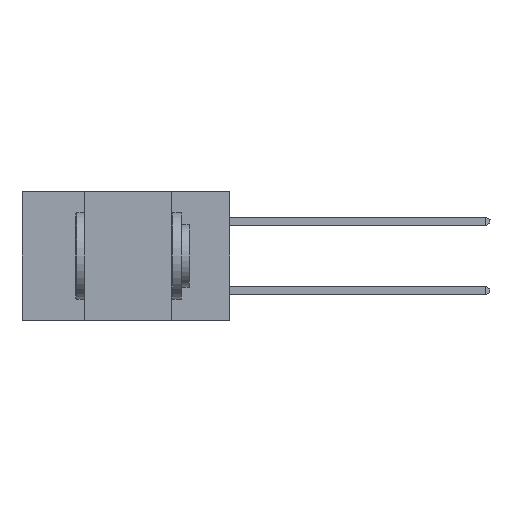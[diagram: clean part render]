
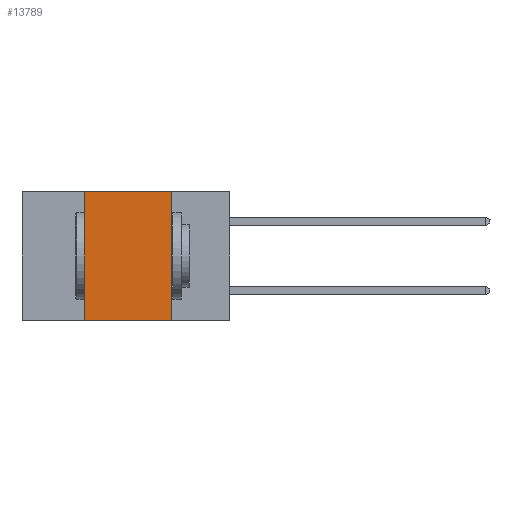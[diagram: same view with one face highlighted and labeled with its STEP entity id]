
A CAD part, left-side view. The second image highlights one B-rep face of the part: STEP entity #13789.
In plain terms, the highlighted planar face has unit normal (-1, 0, 0).
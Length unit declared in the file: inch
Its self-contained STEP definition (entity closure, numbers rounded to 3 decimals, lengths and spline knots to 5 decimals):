
#413 = EDGE_LOOP ( 'NONE', ( #3976, #6658, #12217, #16993 ) ) ;
#875 = LINE ( 'NONE', #3795, #2147 ) ;
#2047 = PLANE ( 'NONE',  #10269 ) ;
#2147 = VECTOR ( 'NONE', #11841, 39.37008 ) ;
#3258 = VERTEX_POINT ( 'NONE', #9242 ) ;
#3274 = CARTESIAN_POINT ( 'NONE',  ( 0., 0.6, 0. ) ) ;
#3795 = CARTESIAN_POINT ( 'NONE',  ( 0., 0.17, -0.37 ) ) ;
#3976 = ORIENTED_EDGE ( 'NONE', *, *, #6549, .F. ) ;
#5056 = EDGE_CURVE ( 'NONE', #7858, #17251, #11684, .T. ) ;
#5085 = VERTEX_POINT ( 'NONE', #14628 ) ;
#5785 = CARTESIAN_POINT ( 'NONE',  ( 0., 0.42, -0.37 ) ) ;
#6549 = EDGE_CURVE ( 'NONE', #17251, #5085, #875, .T. ) ;
#6658 = ORIENTED_EDGE ( 'NONE', *, *, #5056, .F. ) ;
#7161 = DIRECTION ( 'NONE',  ( 0., 0., 1. ) ) ;
#7631 = CARTESIAN_POINT ( 'NONE',  ( 0., 0.6, 0. ) ) ;
#7858 = VERTEX_POINT ( 'NONE', #12988 ) ;
#7904 = VECTOR ( 'NONE', #13191, 39.37008 ) ;
#8482 = VECTOR ( 'NONE', #10405, 39.37008 ) ;
#8838 = CARTESIAN_POINT ( 'NONE',  ( 0., 0.17, 0. ) ) ;
#9242 = CARTESIAN_POINT ( 'NONE',  ( 0., 0.42, -0.37 ) ) ;
#10114 = EDGE_CURVE ( 'NONE', #3258, #5085, #14468, .T. ) ;
#10263 = LINE ( 'NONE', #5785, #15673 ) ;
#10269 = AXIS2_PLACEMENT_3D ( 'NONE', #7631, #15756, #11819 ) ;
#10405 = DIRECTION ( 'NONE',  ( 0., -1., 0. ) ) ;
#11684 = LINE ( 'NONE', #3274, #8482 ) ;
#11819 = DIRECTION ( 'NONE',  ( 0., 0., -1. ) ) ;
#11841 = DIRECTION ( 'NONE',  ( 0., 0., -1. ) ) ;
#12217 = ORIENTED_EDGE ( 'NONE', *, *, #14769, .F. ) ;
#12988 = CARTESIAN_POINT ( 'NONE',  ( 0., 0.42, 0. ) ) ;
#13191 = DIRECTION ( 'NONE',  ( 0., -1., 0. ) ) ;
#13789 = ADVANCED_FACE ( 'NONE', ( #14565 ), #2047, .F. ) ;
#14201 = CARTESIAN_POINT ( 'NONE',  ( 0., 0.6, -0.37 ) ) ;
#14468 = LINE ( 'NONE', #14201, #7904 ) ;
#14565 = FACE_OUTER_BOUND ( 'NONE', #413, .T. ) ;
#14628 = CARTESIAN_POINT ( 'NONE',  ( 0., 0.17, -0.37 ) ) ;
#14769 = EDGE_CURVE ( 'NONE', #3258, #7858, #10263, .T. ) ;
#15673 = VECTOR ( 'NONE', #7161, 39.37008 ) ;
#15756 = DIRECTION ( 'NONE',  ( 1., 0., 0. ) ) ;
#16993 = ORIENTED_EDGE ( 'NONE', *, *, #10114, .T. ) ;
#17251 = VERTEX_POINT ( 'NONE', #8838 ) ;
